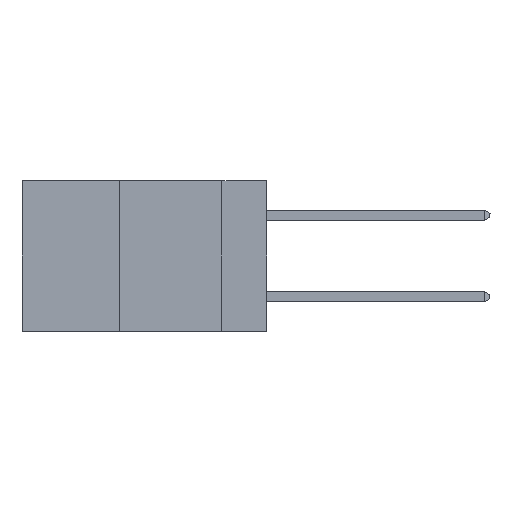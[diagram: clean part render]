
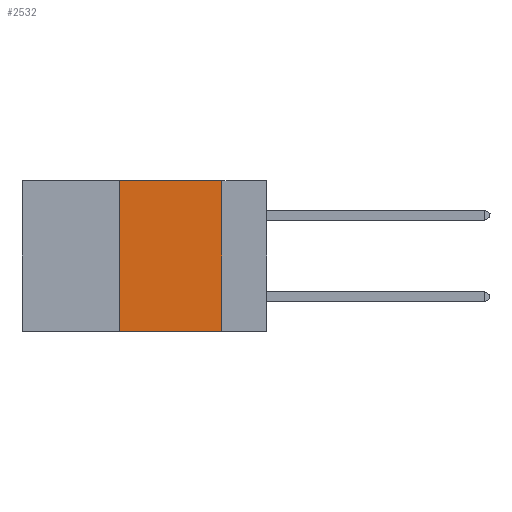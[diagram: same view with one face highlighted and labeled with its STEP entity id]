
A CAD part, left-side view. The second image highlights one B-rep face of the part: STEP entity #2532.
In plain terms, the highlighted planar face has unit normal (-1, 0, 0).
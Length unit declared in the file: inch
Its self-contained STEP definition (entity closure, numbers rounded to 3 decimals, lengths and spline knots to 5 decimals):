
#870 = AXIS2_PLACEMENT_3D ( 'NONE', #9963, #20898, #25402 ) ;
#1067 = VERTEX_POINT ( 'NONE', #9231 ) ;
#1469 = CARTESIAN_POINT ( 'NONE',  ( 0., 0.11, 0. ) ) ;
#1631 = EDGE_CURVE ( 'NONE', #1067, #27774, #19009, .T. ) ;
#1766 = LINE ( 'NONE', #1469, #25279 ) ;
#2532 = ADVANCED_FACE ( 'NONE', ( #23285 ), #2762, .F. ) ;
#2762 = PLANE ( 'NONE',  #870 ) ;
#3285 = ORIENTED_EDGE ( 'NONE', *, *, #26237, .F. ) ;
#3663 = CARTESIAN_POINT ( 'NONE',  ( 0., 0.11, 0. ) ) ;
#5528 = DIRECTION ( 'NONE',  ( 0., 0., 1. ) ) ;
#7107 = EDGE_CURVE ( 'NONE', #1067, #17957, #24794, .T. ) ;
#7313 = EDGE_CURVE ( 'NONE', #27774, #13820, #14749, .T. ) ;
#7492 = VECTOR ( 'NONE', #18032, 39.37008 ) ;
#9231 = CARTESIAN_POINT ( 'NONE',  ( 0., 0.36, -0.37 ) ) ;
#9963 = CARTESIAN_POINT ( 'NONE',  ( 0., 0.6, 0. ) ) ;
#10686 = DIRECTION ( 'NONE',  ( 0., -1., 0. ) ) ;
#10875 = CARTESIAN_POINT ( 'NONE',  ( 0., 0.6, -0.37 ) ) ;
#11902 = ORIENTED_EDGE ( 'NONE', *, *, #7313, .F. ) ;
#13820 = VERTEX_POINT ( 'NONE', #3663 ) ;
#14749 = LINE ( 'NONE', #28544, #28104 ) ;
#15880 = EDGE_LOOP ( 'NONE', ( #3285, #11902, #25834, #17189 ) ) ;
#16008 = CARTESIAN_POINT ( 'NONE',  ( 0., 0.11, -0.37 ) ) ;
#17189 = ORIENTED_EDGE ( 'NONE', *, *, #7107, .T. ) ;
#17957 = VERTEX_POINT ( 'NONE', #16008 ) ;
#18032 = DIRECTION ( 'NONE',  ( 0., -1., 0. ) ) ;
#19009 = LINE ( 'NONE', #21702, #19828 ) ;
#19828 = VECTOR ( 'NONE', #5528, 39.37008 ) ;
#20898 = DIRECTION ( 'NONE',  ( 1., 0., 0. ) ) ;
#21702 = CARTESIAN_POINT ( 'NONE',  ( 0., 0.36, 0. ) ) ;
#23175 = CARTESIAN_POINT ( 'NONE',  ( 0., 0.36, 0. ) ) ;
#23285 = FACE_OUTER_BOUND ( 'NONE', #15880, .T. ) ;
#24098 = DIRECTION ( 'NONE',  ( 0., 0., -1. ) ) ;
#24794 = LINE ( 'NONE', #10875, #7492 ) ;
#25279 = VECTOR ( 'NONE', #24098, 39.37008 ) ;
#25402 = DIRECTION ( 'NONE',  ( 0., 0., -1. ) ) ;
#25834 = ORIENTED_EDGE ( 'NONE', *, *, #1631, .F. ) ;
#26237 = EDGE_CURVE ( 'NONE', #13820, #17957, #1766, .T. ) ;
#27774 = VERTEX_POINT ( 'NONE', #23175 ) ;
#28104 = VECTOR ( 'NONE', #10686, 39.37008 ) ;
#28544 = CARTESIAN_POINT ( 'NONE',  ( 0., 0.6, 0. ) ) ;
